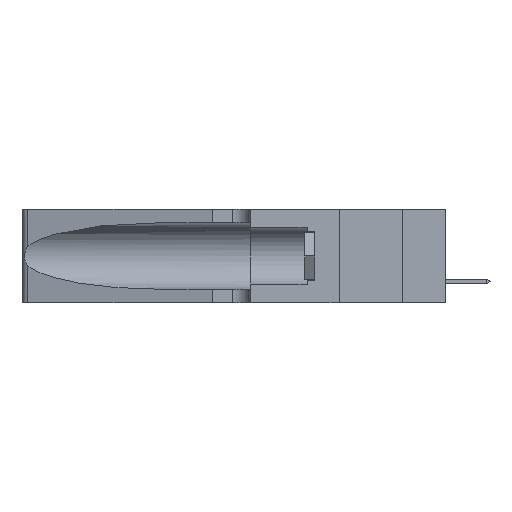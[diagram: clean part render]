
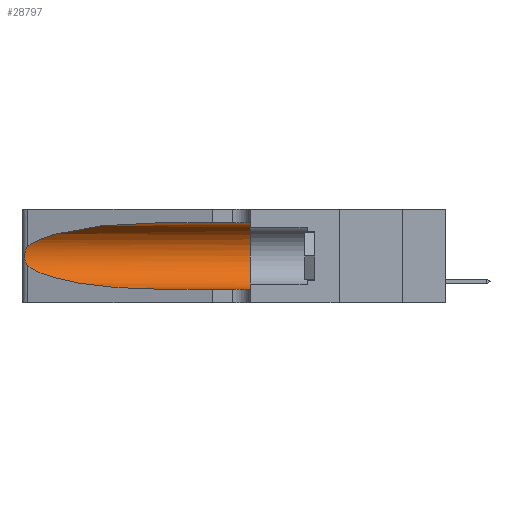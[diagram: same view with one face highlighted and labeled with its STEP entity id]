
A CAD part, left-side view. The second image highlights one B-rep face of the part: STEP entity #28797.
In plain terms, the highlighted cylindrical face has radius 3.308 mm (diameter 6.617 mm), a partial arc.
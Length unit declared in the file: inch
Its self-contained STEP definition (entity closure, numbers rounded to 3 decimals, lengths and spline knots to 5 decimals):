
#318 = ORIENTED_EDGE ( 'NONE', *, *, #46020, .F. ) ;
#448 = CARTESIAN_POINT ( 'NONE',  ( 0.26018, 1.23835, 0.19895 ) ) ;
#1040 = CARTESIAN_POINT ( 'NONE',  ( 0.1305, 0.35, 0.31525 ) ) ;
#1738 = CARTESIAN_POINT ( 'NONE',  ( 0.25789, 1.23486, 0.15765 ) ) ;
#2208 = VERTEX_POINT ( 'NONE', #31890 ) ;
#3987 = DIRECTION ( 'NONE',  ( 0., -1., 0. ) ) ;
#4284 = CARTESIAN_POINT ( 'NONE',  ( 0.25487, 1.22718, 0.22369 ) ) ;
#4532 = CARTESIAN_POINT ( 'NONE',  ( 0.25639, 1.23184, 0.21858 ) ) ;
#7523 = ORIENTED_EDGE ( 'NONE', *, *, #41831, .F. ) ;
#7578 = EDGE_CURVE ( 'NONE', #2208, #22026, #14918, .T. ) ;
#7731 = AXIS2_PLACEMENT_3D ( 'NONE', #46600, #23946, #12756 ) ;
#8050 = CARTESIAN_POINT ( 'NONE',  ( 0.18966, 0.96281, 0.05475 ) ) ;
#8382 = VERTEX_POINT ( 'NONE', #28466 ) ;
#8948 = CARTESIAN_POINT ( 'NONE',  ( 0.26075, 1.23896, 0.178 ) ) ;
#9139 = ORIENTED_EDGE ( 'NONE', *, *, #29633, .T. ) ;
#11687 = CARTESIAN_POINT ( 'NONE',  ( 0.1305, 1.61858, 0.31525 ) ) ;
#12366 = EDGE_CURVE ( 'NONE', #22026, #42945, #33273, .T. ) ;
#12756 = DIRECTION ( 'NONE',  ( 0., 0., -1. ) ) ;
#14053 = AXIS2_PLACEMENT_3D ( 'NONE', #45453, #41556, #18820 ) ;
#14075 = ORIENTED_EDGE ( 'NONE', *, *, #12366, .T. ) ;
#14295 = CARTESIAN_POINT ( 'NONE',  ( 0.25555, 1.22994, 0.2215 ) ) ;
#14814 = VECTOR ( 'NONE', #3987, 39.37008 ) ;
#14918 =( BOUNDED_CURVE ( )  B_SPLINE_CURVE ( 3, ( #19840, #46326, #8050, #27314 ),
 .UNSPECIFIED., .F., .F. ) 
 B_SPLINE_CURVE_WITH_KNOTS ( ( 4, 4 ),
 ( 3.44316, 4.71239 ),
 .UNSPECIFIED. ) 
 CURVE ( )  GEOMETRIC_REPRESENTATION_ITEM ( )  RATIONAL_B_SPLINE_CURVE ( ( 1., 0.87, 0.87, 1. ) ) 
 REPRESENTATION_ITEM ( '' )  );
#15414 = CARTESIAN_POINT ( 'NONE',  ( 0.25787, 1.23484, 0.2124 ) ) ;
#18198 = EDGE_LOOP ( 'NONE', ( #23073, #9139, #40970, #14075, #318, #7523 ) ) ;
#18820 = DIRECTION ( 'NONE',  ( 0., 0., 1. ) ) ;
#19840 = CARTESIAN_POINT ( 'NONE',  ( 0.25487, 1.22718, 0.14631 ) ) ;
#20439 = CARTESIAN_POINT ( 'NONE',  ( 0.26017, 1.23833, 0.17102 ) ) ;
#21294 = CARTESIAN_POINT ( 'NONE',  ( 0.25555, 1.22993, 0.14849 ) ) ;
#21561 = VERTEX_POINT ( 'NONE', #1040 ) ;
#22026 = VERTEX_POINT ( 'NONE', #24320 ) ;
#22944 = CARTESIAN_POINT ( 'NONE',  ( 0.25854, 1.2359, 0.20912 ) ) ;
#23073 = ORIENTED_EDGE ( 'NONE', *, *, #41747, .T. ) ;
#23353 = CARTESIAN_POINT ( 'NONE',  ( 0.25487, 1.22718, 0.22369 ) ) ;
#23946 = DIRECTION ( 'NONE',  ( 0., -1., 0. ) ) ;
#24320 = CARTESIAN_POINT ( 'NONE',  ( 0.1305, 0.72297, 0.05475 ) ) ;
#24488 = CARTESIAN_POINT ( 'NONE',  ( 0.25487, 1.22718, 0.22369 ) ) ;
#27314 = CARTESIAN_POINT ( 'NONE',  ( 0.1305, 0.72297, 0.05475 ) ) ;
#28466 = CARTESIAN_POINT ( 'NONE',  ( 0.1305, 0.72297, 0.31525 ) ) ;
#28603 = FACE_OUTER_BOUND ( 'NONE', #18198, .T. ) ;
#28797 = ADVANCED_FACE ( 'NONE', ( #28603 ), #47529, .F. ) ;
#29633 = EDGE_CURVE ( 'NONE', #48017, #2208, #46359, .T. ) ;
#30850 = VECTOR ( 'NONE', #42313, 39.37008 ) ;
#31176 = CARTESIAN_POINT ( 'NONE',  ( 0.2373, 1.15595, 0.28018 ) ) ;
#31890 = CARTESIAN_POINT ( 'NONE',  ( 0.25487, 1.22718, 0.14631 ) ) ;
#33273 = LINE ( 'NONE', #33624, #30850 ) ;
#33624 = CARTESIAN_POINT ( 'NONE',  ( 0.1305, 1.61858, 0.05475 ) ) ;
#34442 = CARTESIAN_POINT ( 'NONE',  ( 0.26075, 1.23896, 0.19203 ) ) ;
#36103 = CARTESIAN_POINT ( 'NONE',  ( 0.25639, 1.23186, 0.15144 ) ) ;
#36724 = LINE ( 'NONE', #11687, #14814 ) ;
#37867 = CARTESIAN_POINT ( 'NONE',  ( 0.25487, 1.22718, 0.14631 ) ) ;
#38637 = CARTESIAN_POINT ( 'NONE',  ( 0.18966, 0.96281, 0.31525 ) ) ;
#38874 =( BOUNDED_CURVE ( )  B_SPLINE_CURVE ( 3, ( #41959, #38637, #31176, #4284 ),
 .UNSPECIFIED., .F., .F. ) 
 B_SPLINE_CURVE_WITH_KNOTS ( ( 4, 4 ),
 ( 1.5708, 2.84003 ),
 .UNSPECIFIED. ) 
 CURVE ( )  GEOMETRIC_REPRESENTATION_ITEM ( )  RATIONAL_B_SPLINE_CURVE ( ( 1., 0.87, 0.87, 1. ) ) 
 REPRESENTATION_ITEM ( '' )  );
#40970 = ORIENTED_EDGE ( 'NONE', *, *, #7578, .T. ) ;
#41556 = DIRECTION ( 'NONE',  ( 0., 1., 0. ) ) ;
#41747 = EDGE_CURVE ( 'NONE', #8382, #48017, #38874, .T. ) ;
#41831 = EDGE_CURVE ( 'NONE', #8382, #21561, #36724, .T. ) ;
#41959 = CARTESIAN_POINT ( 'NONE',  ( 0.1305, 0.72297, 0.31525 ) ) ;
#42313 = DIRECTION ( 'NONE',  ( 0., -1., 0. ) ) ;
#42945 = VERTEX_POINT ( 'NONE', #44609 ) ;
#43000 = CARTESIAN_POINT ( 'NONE',  ( 0.25856, 1.23593, 0.16098 ) ) ;
#43938 = CIRCLE ( 'NONE', #14053, 0.13025 ) ;
#44609 = CARTESIAN_POINT ( 'NONE',  ( 0.1305, 0.35, 0.05475 ) ) ;
#45453 = CARTESIAN_POINT ( 'NONE',  ( 0.1305, 0.35, 0.185 ) ) ;
#46020 = EDGE_CURVE ( 'NONE', #21561, #42945, #43938, .T. ) ;
#46326 = CARTESIAN_POINT ( 'NONE',  ( 0.2373, 1.15595, 0.08982 ) ) ;
#46359 = B_SPLINE_CURVE_WITH_KNOTS ( 'NONE', 3,
 ( #24488, #14295, #4532, #15414, #22944, #448, #34442, #8948, #20439, #43000, #1738, #36103, #21294, #37867 ),
 .UNSPECIFIED., .F., .F.,
 ( 4, 2, 2, 2, 2, 2, 4 ),
 ( 0., 0.00027, 0.00053, 0.00107, 0.0016, 0.00187, 0.00214 ),
 .UNSPECIFIED. ) ;
#46600 = CARTESIAN_POINT ( 'NONE',  ( 0.1305, 1.61858, 0.185 ) ) ;
#47529 = CYLINDRICAL_SURFACE ( 'NONE', #7731, 0.13025 ) ;
#48017 = VERTEX_POINT ( 'NONE', #23353 ) ;
